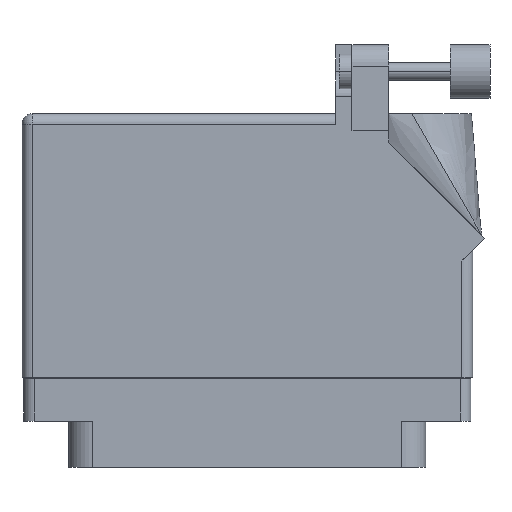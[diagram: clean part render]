
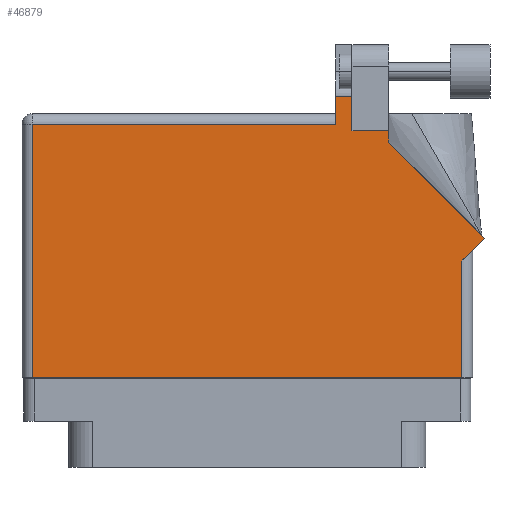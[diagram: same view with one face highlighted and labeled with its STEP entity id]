
A CAD part, front view. The second image highlights one B-rep face of the part: STEP entity #46879.
In plain terms, the highlighted face is planar.
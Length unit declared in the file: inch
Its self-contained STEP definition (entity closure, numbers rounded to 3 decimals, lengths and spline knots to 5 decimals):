
#235 = CARTESIAN_POINT ( 'NONE',  ( 0.82, 1.26442, 0.455 ) ) ;
#802 = VECTOR ( 'NONE', #29106, 39.37008 ) ;
#925 = CARTESIAN_POINT ( 'NONE',  ( 0.82, 1.33, 0.455 ) ) ;
#977 = CARTESIAN_POINT ( 'NONE',  ( 0.607, 1.5315, 0.455 ) ) ;
#1035 = ORIENTED_EDGE ( 'NONE', *, *, #11903, .T. ) ;
#1121 = ORIENTED_EDGE ( 'NONE', *, *, #6924, .T. ) ;
#1670 = PLANE ( 'NONE',  #47153 ) ;
#2545 = EDGE_CURVE ( 'NONE', #13312, #5766, #14198, .T. ) ;
#2633 = CARTESIAN_POINT ( 'NONE',  ( -1.306, 1.368, 0.455 ) ) ;
#2949 = EDGE_LOOP ( 'NONE', ( #15607, #4388, #1035, #1121, #52294, #37281, #39666, #33850, #12397, #15339, #33946 ) ) ;
#3491 = EDGE_CURVE ( 'NONE', #45677, #37826, #40687, .T. ) ;
#3496 = VECTOR ( 'NONE', #9193, 39.37008 ) ;
#4388 = ORIENTED_EDGE ( 'NONE', *, *, #8892, .T. ) ;
#5284 = EDGE_CURVE ( 'NONE', #37826, #6606, #14814, .T. ) ;
#5766 = VERTEX_POINT ( 'NONE', #977 ) ;
#5890 = DIRECTION ( 'NONE',  ( 0., 0., -1. ) ) ;
#6606 = VERTEX_POINT ( 'NONE', #48422 ) ;
#6924 = EDGE_CURVE ( 'NONE', #21005, #32550, #20538, .T. ) ;
#7388 = EDGE_CURVE ( 'NONE', #44126, #36472, #32547, .T. ) ;
#8892 = EDGE_CURVE ( 'NONE', #5766, #32193, #19729, .T. ) ;
#9082 = VECTOR ( 'NONE', #46746, 39.37008 ) ;
#9193 = DIRECTION ( 'NONE',  ( 0., 1., 0. ) ) ;
#10229 = DIRECTION ( 'NONE',  ( 1., 0., 0. ) ) ;
#11630 = VECTOR ( 'NONE', #40177, 39.37008 ) ;
#11903 = EDGE_CURVE ( 'NONE', #32193, #21005, #23684, .T. ) ;
#12397 = ORIENTED_EDGE ( 'NONE', *, *, #21014, .T. ) ;
#13312 = VERTEX_POINT ( 'NONE', #49917 ) ;
#13753 = CARTESIAN_POINT ( 'NONE',  ( 0.513, 1.43, 0.455 ) ) ;
#13771 = CARTESIAN_POINT ( 'NONE',  ( -1.306, 1.43, 0.455 ) ) ;
#14198 = LINE ( 'NONE', #44004, #41454 ) ;
#14814 = LINE ( 'NONE', #24779, #3496 ) ;
#14973 = CARTESIAN_POINT ( 'NONE',  ( -1.244, -0.1, 0.455 ) ) ;
#15249 = LINE ( 'NONE', #45906, #21010 ) ;
#15339 = ORIENTED_EDGE ( 'NONE', *, *, #7388, .T. ) ;
#15607 = ORIENTED_EDGE ( 'NONE', *, *, #2545, .T. ) ;
#16431 = VERTEX_POINT ( 'NONE', #39652 ) ;
#18017 = CARTESIAN_POINT ( 'NONE',  ( -1.306, -0.1, 0.455 ) ) ;
#19729 = LINE ( 'NONE', #49659, #802 ) ;
#20538 = LINE ( 'NONE', #2633, #41447 ) ;
#20858 = DIRECTION ( 'NONE',  ( -1., 0., 0. ) ) ;
#21005 = VERTEX_POINT ( 'NONE', #45725 ) ;
#21010 = VECTOR ( 'NONE', #45192, 39.37008 ) ;
#21014 = EDGE_CURVE ( 'NONE', #16431, #44126, #15249, .T. ) ;
#21990 = DIRECTION ( 'NONE',  ( -1., 0., 0. ) ) ;
#23684 = LINE ( 'NONE', #13753, #9082 ) ;
#24331 = DIRECTION ( 'NONE',  ( -1., 0., 0. ) ) ;
#24395 = EDGE_CURVE ( 'NONE', #32550, #45677, #52256, .T. ) ;
#24779 = CARTESIAN_POINT ( 'NONE',  ( 1.244, 0.637, 0.455 ) ) ;
#24908 = CARTESIAN_POINT ( 'NONE',  ( -1.244, -0.1, 0.455 ) ) ;
#25102 = CARTESIAN_POINT ( 'NONE',  ( 1.244, -0.1, 0.455 ) ) ;
#25838 = CARTESIAN_POINT ( 'NONE',  ( -1.244, 1.368, 0.455 ) ) ;
#27179 = VECTOR ( 'NONE', #20858, 39.37008 ) ;
#28287 = CARTESIAN_POINT ( 'NONE',  ( 0.82, 1.33, 0.455 ) ) ;
#29106 = DIRECTION ( 'NONE',  ( -1., 0., 0. ) ) ;
#30369 = DIRECTION ( 'NONE',  ( 0.707, 0.707, 0. ) ) ;
#32072 = VECTOR ( 'NONE', #30369, 39.37008 ) ;
#32193 = VERTEX_POINT ( 'NONE', #45920 ) ;
#32539 = FACE_OUTER_BOUND ( 'NONE', #2949, .T. ) ;
#32547 = LINE ( 'NONE', #235, #11630 ) ;
#32550 = VERTEX_POINT ( 'NONE', #25838 ) ;
#32898 = DIRECTION ( 'NONE',  ( 0., -1., 0. ) ) ;
#33850 = ORIENTED_EDGE ( 'NONE', *, *, #45129, .T. ) ;
#33891 = VECTOR ( 'NONE', #32898, 39.37008 ) ;
#33899 = CARTESIAN_POINT ( 'NONE',  ( 1.306, 0.637, 0.455 ) ) ;
#33946 = ORIENTED_EDGE ( 'NONE', *, *, #39221, .T. ) ;
#36472 = VERTEX_POINT ( 'NONE', #28287 ) ;
#37281 = ORIENTED_EDGE ( 'NONE', *, *, #3491, .T. ) ;
#37826 = VERTEX_POINT ( 'NONE', #25102 ) ;
#38803 = VECTOR ( 'NONE', #10229, 39.37008 ) ;
#39221 = EDGE_CURVE ( 'NONE', #36472, #13312, #45584, .T. ) ;
#39652 = CARTESIAN_POINT ( 'NONE',  ( 1.37671, 0.70771, 0.455 ) ) ;
#39666 = ORIENTED_EDGE ( 'NONE', *, *, #5284, .T. ) ;
#40177 = DIRECTION ( 'NONE',  ( 0., 1., 0. ) ) ;
#40687 = LINE ( 'NONE', #18017, #38803 ) ;
#41447 = VECTOR ( 'NONE', #24331, 39.37008 ) ;
#41454 = VECTOR ( 'NONE', #48048, 39.37008 ) ;
#41856 = CARTESIAN_POINT ( 'NONE',  ( 0.82, 1.26442, 0.455 ) ) ;
#42821 = LINE ( 'NONE', #33899, #32072 ) ;
#44004 = CARTESIAN_POINT ( 'NONE',  ( 0.607, 1.33, 0.455 ) ) ;
#44126 = VERTEX_POINT ( 'NONE', #41856 ) ;
#45129 = EDGE_CURVE ( 'NONE', #6606, #16431, #42821, .T. ) ;
#45192 = DIRECTION ( 'NONE',  ( -0.707, 0.707, 0. ) ) ;
#45584 = LINE ( 'NONE', #925, #27179 ) ;
#45677 = VERTEX_POINT ( 'NONE', #14973 ) ;
#45725 = CARTESIAN_POINT ( 'NONE',  ( 0.513, 1.368, 0.455 ) ) ;
#45906 = CARTESIAN_POINT ( 'NONE',  ( 1.37671, 0.70771, 0.455 ) ) ;
#45920 = CARTESIAN_POINT ( 'NONE',  ( 0.513, 1.5315, 0.455 ) ) ;
#46746 = DIRECTION ( 'NONE',  ( 0., -1., 0. ) ) ;
#46879 = ADVANCED_FACE ( 'NONE', ( #32539 ), #1670, .F. ) ;
#47153 = AXIS2_PLACEMENT_3D ( 'NONE', #13771, #5890, #21990 ) ;
#48048 = DIRECTION ( 'NONE',  ( 0., 1., 0. ) ) ;
#48422 = CARTESIAN_POINT ( 'NONE',  ( 1.244, 0.575, 0.455 ) ) ;
#49659 = CARTESIAN_POINT ( 'NONE',  ( 0.93777, 1.5315, 0.455 ) ) ;
#49917 = CARTESIAN_POINT ( 'NONE',  ( 0.607, 1.33, 0.455 ) ) ;
#52256 = LINE ( 'NONE', #24908, #33891 ) ;
#52294 = ORIENTED_EDGE ( 'NONE', *, *, #24395, .T. ) ;
